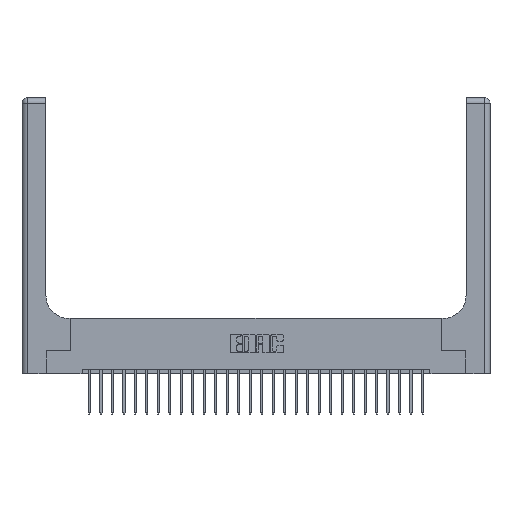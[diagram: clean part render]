
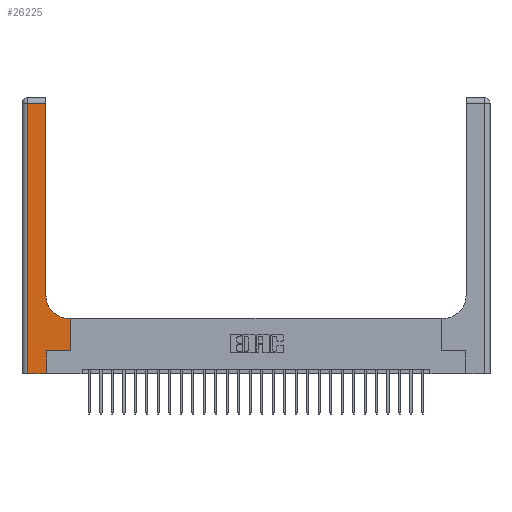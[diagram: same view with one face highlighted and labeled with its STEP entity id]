
A CAD part, top view. The second image highlights one B-rep face of the part: STEP entity #26225.
In plain terms, the highlighted planar face has unit normal (0, 0, 1).
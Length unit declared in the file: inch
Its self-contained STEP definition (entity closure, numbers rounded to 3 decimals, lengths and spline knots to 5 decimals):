
#212 = LINE ( 'NONE', #26328, #10057 ) ;
#425 = VECTOR ( 'NONE', #7582, 39.37008 ) ;
#630 = ORIENTED_EDGE ( 'NONE', *, *, #13606, .T. ) ;
#887 = CARTESIAN_POINT ( 'NONE',  ( 0., 2.94, 0.37 ) ) ;
#1635 = CARTESIAN_POINT ( 'NONE',  ( 0.51, 0.85, 0.37 ) ) ;
#2162 = VERTEX_POINT ( 'NONE', #19497 ) ;
#2419 = DIRECTION ( 'NONE',  ( 1., 0., 0. ) ) ;
#2716 = CARTESIAN_POINT ( 'NONE',  ( 0.265, 0., 0.37 ) ) ;
#2790 = VERTEX_POINT ( 'NONE', #24101 ) ;
#2852 = CARTESIAN_POINT ( 'NONE',  ( 0.06, 0., 0.37 ) ) ;
#3135 = CARTESIAN_POINT ( 'NONE',  ( 0.26, 3., 0.37 ) ) ;
#3283 = ORIENTED_EDGE ( 'NONE', *, *, #19160, .T. ) ;
#3534 = EDGE_CURVE ( 'NONE', #2790, #13371, #18242, .T. ) ;
#3767 = VECTOR ( 'NONE', #7906, 39.37008 ) ;
#4003 = EDGE_LOOP ( 'NONE', ( #13068, #4867, #630, #10111, #11004, #15004, #21121, #3283, #23504 ) ) ;
#4867 = ORIENTED_EDGE ( 'NONE', *, *, #3534, .T. ) ;
#5242 = DIRECTION ( 'NONE',  ( 0., 1., 0. ) ) ;
#5683 = LINE ( 'NONE', #6616, #19736 ) ;
#5849 = LINE ( 'NONE', #20684, #5884 ) ;
#5884 = VECTOR ( 'NONE', #8846, 39.37008 ) ;
#6269 = AXIS2_PLACEMENT_3D ( 'NONE', #16172, #8063, #9898 ) ;
#6469 = EDGE_CURVE ( 'NONE', #19008, #20319, #11545, .T. ) ;
#6616 = CARTESIAN_POINT ( 'NONE',  ( 0.265, 0., 0.37 ) ) ;
#6640 = VERTEX_POINT ( 'NONE', #16316 ) ;
#7412 = DIRECTION ( 'NONE',  ( 1., 0., 0. ) ) ;
#7582 = DIRECTION ( 'NONE',  ( 1., 0., 0. ) ) ;
#7791 = PLANE ( 'NONE',  #6269 ) ;
#7906 = DIRECTION ( 'NONE',  ( 0., 1., 0. ) ) ;
#8063 = DIRECTION ( 'NONE',  ( 0., 0., -1. ) ) ;
#8566 = EDGE_CURVE ( 'NONE', #20319, #2162, #5683, .T. ) ;
#8846 = DIRECTION ( 'NONE',  ( 0., -1., 0. ) ) ;
#9898 = DIRECTION ( 'NONE',  ( -1., 0., 0. ) ) ;
#9959 = VECTOR ( 'NONE', #5242, 39.37008 ) ;
#10057 = VECTOR ( 'NONE', #2419, 39.37008 ) ;
#10111 = ORIENTED_EDGE ( 'NONE', *, *, #6469, .T. ) ;
#11004 = ORIENTED_EDGE ( 'NONE', *, *, #8566, .T. ) ;
#11127 = EDGE_CURVE ( 'NONE', #2162, #19420, #212, .T. ) ;
#11545 = LINE ( 'NONE', #23664, #425 ) ;
#11760 = FACE_OUTER_BOUND ( 'NONE', #4003, .T. ) ;
#11963 = VECTOR ( 'NONE', #26198, 39.37008 ) ;
#12082 = CARTESIAN_POINT ( 'NONE',  ( 0.528, 0.25, 0.37 ) ) ;
#12856 = VECTOR ( 'NONE', #19280, 39.37008 ) ;
#13068 = ORIENTED_EDGE ( 'NONE', *, *, #22466, .T. ) ;
#13371 = VERTEX_POINT ( 'NONE', #21939 ) ;
#13606 = EDGE_CURVE ( 'NONE', #13371, #19008, #5849, .T. ) ;
#15004 = ORIENTED_EDGE ( 'NONE', *, *, #11127, .T. ) ;
#15189 = LINE ( 'NONE', #26106, #11963 ) ;
#15422 = LINE ( 'NONE', #3135, #9959 ) ;
#15538 = DIRECTION ( 'NONE',  ( 0., 0., -1. ) ) ;
#16172 = CARTESIAN_POINT ( 'NONE',  ( 0., 3., 0.37 ) ) ;
#16316 = CARTESIAN_POINT ( 'NONE',  ( 0.51, 0.6, 0.37 ) ) ;
#16533 = LINE ( 'NONE', #12082, #3767 ) ;
#16755 = EDGE_CURVE ( 'NONE', #6640, #21192, #16933, .T. ) ;
#16933 = CIRCLE ( 'NONE', #24383, 0.25 ) ;
#17768 = EDGE_CURVE ( 'NONE', #19420, #19816, #16533, .T. ) ;
#18242 = LINE ( 'NONE', #887, #12856 ) ;
#19008 = VERTEX_POINT ( 'NONE', #2852 ) ;
#19160 = EDGE_CURVE ( 'NONE', #19816, #6640, #15189, .T. ) ;
#19280 = DIRECTION ( 'NONE',  ( -1., 0., 0. ) ) ;
#19420 = VERTEX_POINT ( 'NONE', #22614 ) ;
#19461 = CARTESIAN_POINT ( 'NONE',  ( 0.528, 0.6, 0.37 ) ) ;
#19497 = CARTESIAN_POINT ( 'NONE',  ( 0.265, 0.25, 0.37 ) ) ;
#19736 = VECTOR ( 'NONE', #25013, 39.37008 ) ;
#19816 = VERTEX_POINT ( 'NONE', #19461 ) ;
#20319 = VERTEX_POINT ( 'NONE', #2716 ) ;
#20684 = CARTESIAN_POINT ( 'NONE',  ( 0.06, 3., 0.37 ) ) ;
#21121 = ORIENTED_EDGE ( 'NONE', *, *, #17768, .T. ) ;
#21192 = VERTEX_POINT ( 'NONE', #22833 ) ;
#21939 = CARTESIAN_POINT ( 'NONE',  ( 0.06, 2.94, 0.37 ) ) ;
#22466 = EDGE_CURVE ( 'NONE', #21192, #2790, #15422, .T. ) ;
#22614 = CARTESIAN_POINT ( 'NONE',  ( 0.528, 0.25, 0.37 ) ) ;
#22833 = CARTESIAN_POINT ( 'NONE',  ( 0.26, 0.85, 0.37 ) ) ;
#23504 = ORIENTED_EDGE ( 'NONE', *, *, #16755, .T. ) ;
#23664 = CARTESIAN_POINT ( 'NONE',  ( 0., 0., 0.37 ) ) ;
#24101 = CARTESIAN_POINT ( 'NONE',  ( 0.26, 2.94, 0.37 ) ) ;
#24383 = AXIS2_PLACEMENT_3D ( 'NONE', #1635, #15538, #7412 ) ;
#25013 = DIRECTION ( 'NONE',  ( 0., 1., 0. ) ) ;
#26106 = CARTESIAN_POINT ( 'NONE',  ( 0.26, 0.6, 0.37 ) ) ;
#26198 = DIRECTION ( 'NONE',  ( -1., 0., 0. ) ) ;
#26225 = ADVANCED_FACE ( 'NONE', ( #11760 ), #7791, .F. ) ;
#26328 = CARTESIAN_POINT ( 'NONE',  ( 0.265, 0.25, 0.37 ) ) ;
